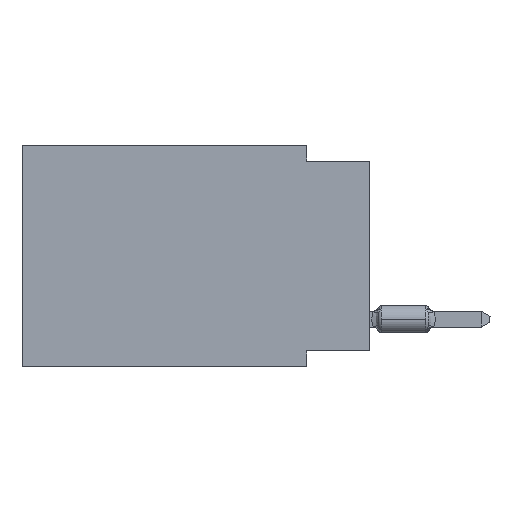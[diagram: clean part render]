
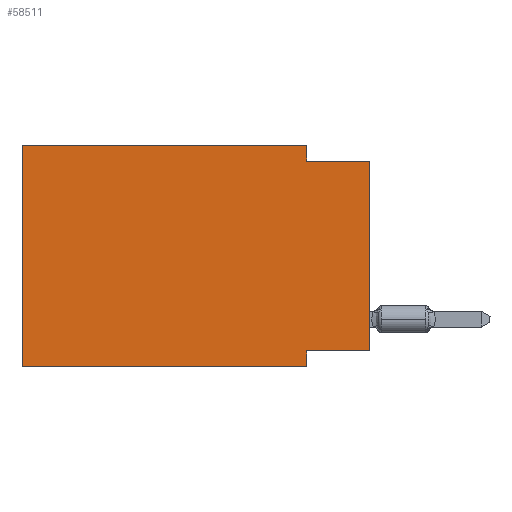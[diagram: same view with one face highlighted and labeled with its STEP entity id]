
A CAD part, left-side view. The second image highlights one B-rep face of the part: STEP entity #58511.
In plain terms, the highlighted planar face has unit normal (-1, 0, 0).
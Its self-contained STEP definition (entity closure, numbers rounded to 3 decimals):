
#995 = VECTOR ( 'NONE', #30182, 1000. ) ;
#3319 = EDGE_CURVE ( 'NONE', #25591, #7138, #41240, .T. ) ;
#3440 = VECTOR ( 'NONE', #16599, 1000. ) ;
#4013 = VERTEX_POINT ( 'NONE', #60793 ) ;
#7138 = VERTEX_POINT ( 'NONE', #13478 ) ;
#7225 = LINE ( 'NONE', #17958, #7352 ) ;
#7352 = VECTOR ( 'NONE', #7544, 1000. ) ;
#7544 = DIRECTION ( 'NONE',  ( 0., 0., -1. ) ) ;
#9206 = EDGE_CURVE ( 'NONE', #64504, #57238, #33555, .T. ) ;
#9441 = LINE ( 'NONE', #55691, #995 ) ;
#13478 = CARTESIAN_POINT ( 'NONE',  ( 0., 2.54, -8.89 ) ) ;
#13791 = ORIENTED_EDGE ( 'NONE', *, *, #35655, .F. ) ;
#13803 = CARTESIAN_POINT ( 'NONE',  ( 0., 0., -0.635 ) ) ;
#15362 = VERTEX_POINT ( 'NONE', #49064 ) ;
#15385 = ORIENTED_EDGE ( 'NONE', *, *, #41862, .F. ) ;
#15592 = VECTOR ( 'NONE', #17044, 1000. ) ;
#16599 = DIRECTION ( 'NONE',  ( 0., -1., 0. ) ) ;
#17044 = DIRECTION ( 'NONE',  ( 0., 0., 1. ) ) ;
#17958 = CARTESIAN_POINT ( 'NONE',  ( 0., 2.54, 0. ) ) ;
#23512 = VECTOR ( 'NONE', #39271, 1000. ) ;
#23650 = LINE ( 'NONE', #55167, #32348 ) ;
#24746 = VERTEX_POINT ( 'NONE', #42837 ) ;
#25591 = VERTEX_POINT ( 'NONE', #42599 ) ;
#25765 = DIRECTION ( 'NONE',  ( 1., 0., 0. ) ) ;
#25796 = DIRECTION ( 'NONE',  ( 0., 0., -1. ) ) ;
#26100 = FACE_OUTER_BOUND ( 'NONE', #31869, .T. ) ;
#28248 = EDGE_CURVE ( 'NONE', #24746, #57238, #32118, .T. ) ;
#30182 = DIRECTION ( 'NONE',  ( 0., -1., 0. ) ) ;
#30506 = CARTESIAN_POINT ( 'NONE',  ( 0., 2.54, -8.89 ) ) ;
#31869 = EDGE_LOOP ( 'NONE', ( #66118, #46255, #62496, #42701, #13791, #63228, #62017, #15385 ) ) ;
#32015 = LINE ( 'NONE', #62508, #3440 ) ;
#32118 = LINE ( 'NONE', #53563, #15592 ) ;
#32145 = PLANE ( 'NONE',  #57018 ) ;
#32267 = EDGE_CURVE ( 'NONE', #4013, #7138, #9441, .T. ) ;
#32348 = VECTOR ( 'NONE', #35039, 1000. ) ;
#33406 = EDGE_CURVE ( 'NONE', #15362, #64504, #7225, .T. ) ;
#33555 = LINE ( 'NONE', #13803, #23512 ) ;
#35039 = DIRECTION ( 'NONE',  ( 0., 1., 0. ) ) ;
#35655 = EDGE_CURVE ( 'NONE', #4013, #55938, #48269, .T. ) ;
#36828 = CARTESIAN_POINT ( 'NONE',  ( 0., 0., -0.635 ) ) ;
#39271 = DIRECTION ( 'NONE',  ( 0., -1., 0. ) ) ;
#41240 = LINE ( 'NONE', #30506, #51888 ) ;
#41437 = EDGE_CURVE ( 'NONE', #55938, #15362, #32015, .T. ) ;
#41847 = CARTESIAN_POINT ( 'NONE',  ( 0., 13.97, 0. ) ) ;
#41862 = EDGE_CURVE ( 'NONE', #24746, #25591, #23650, .T. ) ;
#41865 = DIRECTION ( 'NONE',  ( 0., 0., -1. ) ) ;
#42599 = CARTESIAN_POINT ( 'NONE',  ( 0., 2.54, -8.255 ) ) ;
#42701 = ORIENTED_EDGE ( 'NONE', *, *, #41437, .F. ) ;
#42837 = CARTESIAN_POINT ( 'NONE',  ( 0., 0., -8.255 ) ) ;
#46255 = ORIENTED_EDGE ( 'NONE', *, *, #9206, .F. ) ;
#46571 = CARTESIAN_POINT ( 'NONE',  ( 0., 13.97, 0. ) ) ;
#48269 = LINE ( 'NONE', #49272, #55882 ) ;
#49064 = CARTESIAN_POINT ( 'NONE',  ( 0., 2.54, 0. ) ) ;
#49272 = CARTESIAN_POINT ( 'NONE',  ( 0., 13.97, 0. ) ) ;
#51888 = VECTOR ( 'NONE', #25796, 1000. ) ;
#53563 = CARTESIAN_POINT ( 'NONE',  ( 0., 0., 0. ) ) ;
#55167 = CARTESIAN_POINT ( 'NONE',  ( 0., 0., -8.255 ) ) ;
#55691 = CARTESIAN_POINT ( 'NONE',  ( 0., 13.97, -8.89 ) ) ;
#55882 = VECTOR ( 'NONE', #59321, 1000. ) ;
#55938 = VERTEX_POINT ( 'NONE', #41847 ) ;
#57018 = AXIS2_PLACEMENT_3D ( 'NONE', #46571, #25765, #41865 ) ;
#57238 = VERTEX_POINT ( 'NONE', #36828 ) ;
#58511 = ADVANCED_FACE ( 'NONE', ( #26100 ), #32145, .F. ) ;
#59321 = DIRECTION ( 'NONE',  ( 0., 0., 1. ) ) ;
#60793 = CARTESIAN_POINT ( 'NONE',  ( 0., 13.97, -8.89 ) ) ;
#60831 = CARTESIAN_POINT ( 'NONE',  ( 0., 2.54, -0.635 ) ) ;
#62017 = ORIENTED_EDGE ( 'NONE', *, *, #3319, .F. ) ;
#62496 = ORIENTED_EDGE ( 'NONE', *, *, #33406, .F. ) ;
#62508 = CARTESIAN_POINT ( 'NONE',  ( 0., 13.97, 0. ) ) ;
#63228 = ORIENTED_EDGE ( 'NONE', *, *, #32267, .T. ) ;
#64504 = VERTEX_POINT ( 'NONE', #60831 ) ;
#66118 = ORIENTED_EDGE ( 'NONE', *, *, #28248, .T. ) ;
